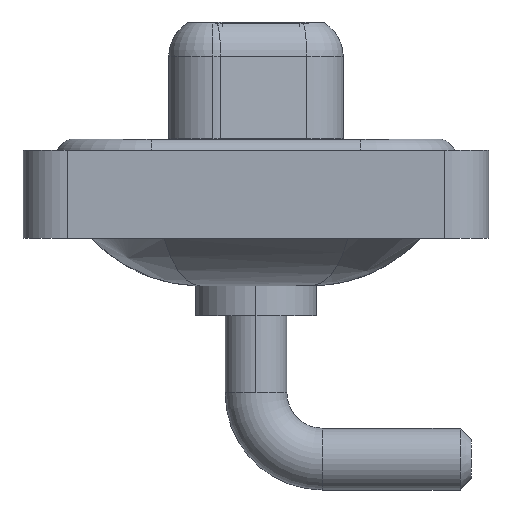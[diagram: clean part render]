
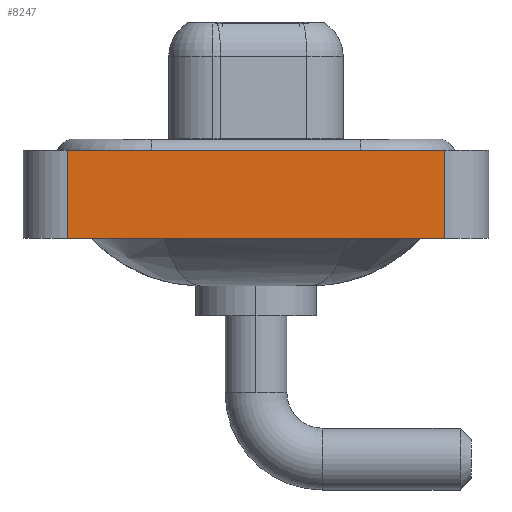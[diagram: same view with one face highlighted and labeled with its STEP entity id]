
A CAD part, left-side view. The second image highlights one B-rep face of the part: STEP entity #8247.
In plain terms, the highlighted planar face has unit normal (-1, 0, 0).
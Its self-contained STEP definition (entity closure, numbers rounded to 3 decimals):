
#34 = CARTESIAN_POINT ( 'NONE',  ( -7.3, 8.55, 0.4 ) ) ;
#266 = FACE_OUTER_BOUND ( 'NONE', #10367, .T. ) ;
#757 = CARTESIAN_POINT ( 'NONE',  ( -7.3, -8.55, 0.4 ) ) ;
#1048 = LINE ( 'NONE', #10914, #6473 ) ;
#2205 = CARTESIAN_POINT ( 'NONE',  ( -7.3, -8.55, -3.6 ) ) ;
#3102 = EDGE_CURVE ( 'NONE', #8305, #8877, #10736, .T. ) ;
#3551 = DIRECTION ( 'NONE',  ( 0., -1., 0. ) ) ;
#4010 = PLANE ( 'NONE',  #7683 ) ;
#4489 = CARTESIAN_POINT ( 'NONE',  ( -7.3, 8.55, -3.6 ) ) ;
#4631 = LINE ( 'NONE', #2205, #15555 ) ;
#5599 = LINE ( 'NONE', #9563, #5960 ) ;
#5751 = DIRECTION ( 'NONE',  ( 0., -1., 0. ) ) ;
#5960 = VECTOR ( 'NONE', #8097, 1000. ) ;
#5967 = ORIENTED_EDGE ( 'NONE', *, *, #3102, .T. ) ;
#6445 = ORIENTED_EDGE ( 'NONE', *, *, #11447, .F. ) ;
#6473 = VECTOR ( 'NONE', #5751, 1000. ) ;
#7405 = VERTEX_POINT ( 'NONE', #757 ) ;
#7469 = CARTESIAN_POINT ( 'NONE',  ( -7.3, -8.55, -3.6 ) ) ;
#7683 = AXIS2_PLACEMENT_3D ( 'NONE', #7469, #8936, #12393 ) ;
#8097 = DIRECTION ( 'NONE',  ( 0., 0., 1. ) ) ;
#8247 = ADVANCED_FACE ( 'NONE', ( #266 ), #4010, .T. ) ;
#8305 = VERTEX_POINT ( 'NONE', #4489 ) ;
#8877 = VERTEX_POINT ( 'NONE', #9696 ) ;
#8936 = DIRECTION ( 'NONE',  ( -1., 0., 0. ) ) ;
#9563 = CARTESIAN_POINT ( 'NONE',  ( -7.3, 8.55, -3.6 ) ) ;
#9696 = CARTESIAN_POINT ( 'NONE',  ( -7.3, -8.55, -3.6 ) ) ;
#9699 = CARTESIAN_POINT ( 'NONE',  ( -7.3, -8.55, -3.6 ) ) ;
#9895 = VECTOR ( 'NONE', #3551, 1000. ) ;
#10367 = EDGE_LOOP ( 'NONE', ( #11697, #6445, #13894, #5967 ) ) ;
#10736 = LINE ( 'NONE', #9699, #9895 ) ;
#10914 = CARTESIAN_POINT ( 'NONE',  ( -7.3, -8.55, 0.4 ) ) ;
#11447 = EDGE_CURVE ( 'NONE', #12357, #7405, #1048, .T. ) ;
#11451 = EDGE_CURVE ( 'NONE', #8877, #7405, #4631, .T. ) ;
#11697 = ORIENTED_EDGE ( 'NONE', *, *, #11451, .T. ) ;
#12357 = VERTEX_POINT ( 'NONE', #34 ) ;
#12393 = DIRECTION ( 'NONE',  ( 0., 0., 1. ) ) ;
#13894 = ORIENTED_EDGE ( 'NONE', *, *, #14133, .F. ) ;
#13907 = DIRECTION ( 'NONE',  ( 0., 0., 1. ) ) ;
#14133 = EDGE_CURVE ( 'NONE', #8305, #12357, #5599, .T. ) ;
#15555 = VECTOR ( 'NONE', #13907, 1000. ) ;
